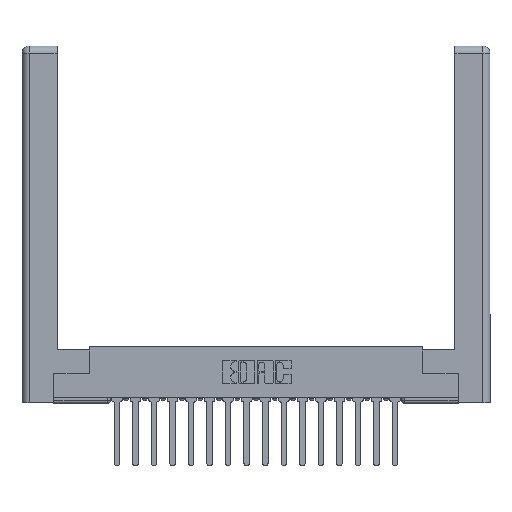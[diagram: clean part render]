
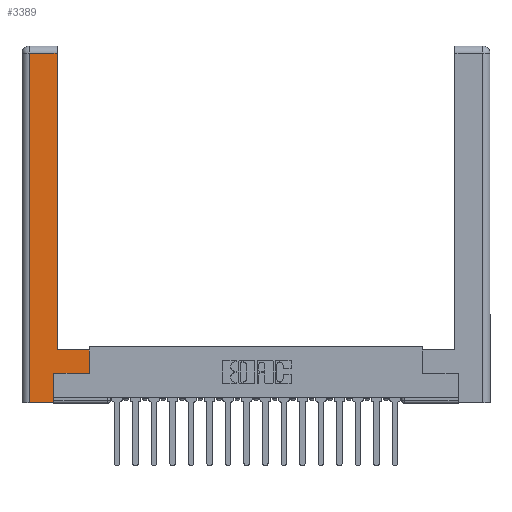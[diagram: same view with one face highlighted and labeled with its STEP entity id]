
A CAD part, top view. The second image highlights one B-rep face of the part: STEP entity #3389.
In plain terms, the highlighted planar face has unit normal (0, 0, 1).
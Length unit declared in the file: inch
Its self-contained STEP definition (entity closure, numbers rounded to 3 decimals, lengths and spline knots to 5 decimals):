
#614 = VECTOR ( 'NONE', #8455, 39.37008 ) ;
#853 = EDGE_CURVE ( 'NONE', #2836, #4499, #2111, .T. ) ;
#856 = EDGE_LOOP ( 'NONE', ( #15141, #6297, #9200, #5167, #18083, #8203, #3710, #19358 ) ) ;
#1286 = DIRECTION ( 'NONE',  ( 0., 1., 0. ) ) ;
#1375 = EDGE_CURVE ( 'NONE', #1869, #11545, #8888, .T. ) ;
#1537 = CARTESIAN_POINT ( 'NONE',  ( 0.565, 0.245, 0. ) ) ;
#1869 = VERTEX_POINT ( 'NONE', #1537 ) ;
#2111 = LINE ( 'NONE', #8160, #614 ) ;
#2508 = CARTESIAN_POINT ( 'NONE',  ( 0.0615, 0., 0. ) ) ;
#2730 = EDGE_CURVE ( 'NONE', #12253, #6543, #13529, .T. ) ;
#2836 = VERTEX_POINT ( 'NONE', #15602 ) ;
#2843 = CARTESIAN_POINT ( 'NONE',  ( 0.565, 0.45, 0. ) ) ;
#2888 = CARTESIAN_POINT ( 'NONE',  ( 0.0615, 2.94, 0. ) ) ;
#3200 = LINE ( 'NONE', #15154, #17868 ) ;
#3276 = EDGE_CURVE ( 'NONE', #8024, #18754, #8373, .T. ) ;
#3389 = ADVANCED_FACE ( 'NONE', ( #11805 ), #5505, .F. ) ;
#3499 = VECTOR ( 'NONE', #13211, 39.37008 ) ;
#3710 = ORIENTED_EDGE ( 'NONE', *, *, #1375, .T. ) ;
#4499 = VERTEX_POINT ( 'NONE', #5431 ) ;
#4807 = DIRECTION ( 'NONE',  ( 1., 0., 0. ) ) ;
#5167 = ORIENTED_EDGE ( 'NONE', *, *, #16092, .T. ) ;
#5282 = CARTESIAN_POINT ( 'NONE',  ( 0.0615, 2.94, 0. ) ) ;
#5431 = CARTESIAN_POINT ( 'NONE',  ( 0.265, 0.245, 0. ) ) ;
#5479 = VECTOR ( 'NONE', #1286, 39.37008 ) ;
#5505 = PLANE ( 'NONE',  #19363 ) ;
#6297 = ORIENTED_EDGE ( 'NONE', *, *, #10881, .T. ) ;
#6543 = VERTEX_POINT ( 'NONE', #16016 ) ;
#7455 = CARTESIAN_POINT ( 'NONE',  ( 0.295, 3., 0. ) ) ;
#7526 = EDGE_CURVE ( 'NONE', #11545, #12253, #13202, .T. ) ;
#8024 = VERTEX_POINT ( 'NONE', #5282 ) ;
#8122 = DIRECTION ( 'NONE',  ( 1., 0., 0. ) ) ;
#8160 = CARTESIAN_POINT ( 'NONE',  ( 0.265, 0.245, 0. ) ) ;
#8203 = ORIENTED_EDGE ( 'NONE', *, *, #19004, .T. ) ;
#8373 = LINE ( 'NONE', #12599, #11798 ) ;
#8455 = DIRECTION ( 'NONE',  ( 0., 1., 0. ) ) ;
#8855 = VECTOR ( 'NONE', #15041, 39.37008 ) ;
#8888 = LINE ( 'NONE', #2843, #3499 ) ;
#9200 = ORIENTED_EDGE ( 'NONE', *, *, #3276, .T. ) ;
#9609 = CARTESIAN_POINT ( 'NONE',  ( 0.295, 0.45, 0. ) ) ;
#10112 = DIRECTION ( 'NONE',  ( -1., 0., 0. ) ) ;
#10156 = CARTESIAN_POINT ( 'NONE',  ( 0.295, 0.45, 0. ) ) ;
#10223 = CARTESIAN_POINT ( 'NONE',  ( 0., 0., 0. ) ) ;
#10576 = VECTOR ( 'NONE', #14580, 39.37008 ) ;
#10881 = EDGE_CURVE ( 'NONE', #6543, #8024, #16418, .T. ) ;
#11545 = VERTEX_POINT ( 'NONE', #17468 ) ;
#11798 = VECTOR ( 'NONE', #14363, 39.37008 ) ;
#11805 = FACE_OUTER_BOUND ( 'NONE', #856, .T. ) ;
#12253 = VERTEX_POINT ( 'NONE', #9609 ) ;
#12599 = CARTESIAN_POINT ( 'NONE',  ( 0.0615, 0., 0. ) ) ;
#12742 = CARTESIAN_POINT ( 'NONE',  ( 0.265, 0., 0. ) ) ;
#13202 = LINE ( 'NONE', #10156, #10576 ) ;
#13211 = DIRECTION ( 'NONE',  ( 0., 1., 0. ) ) ;
#13529 = LINE ( 'NONE', #7455, #5479 ) ;
#14204 = LINE ( 'NONE', #12742, #17138 ) ;
#14363 = DIRECTION ( 'NONE',  ( 0., -1., 0. ) ) ;
#14580 = DIRECTION ( 'NONE',  ( -1., 0., 0. ) ) ;
#14846 = DIRECTION ( 'NONE',  ( 0., 0., -1. ) ) ;
#15041 = DIRECTION ( 'NONE',  ( -1., 0., 0. ) ) ;
#15141 = ORIENTED_EDGE ( 'NONE', *, *, #2730, .T. ) ;
#15154 = CARTESIAN_POINT ( 'NONE',  ( 0.565, 0.245, 0. ) ) ;
#15602 = CARTESIAN_POINT ( 'NONE',  ( 0.265, 0., 0. ) ) ;
#16016 = CARTESIAN_POINT ( 'NONE',  ( 0.295, 2.94, 0. ) ) ;
#16092 = EDGE_CURVE ( 'NONE', #18754, #2836, #14204, .T. ) ;
#16418 = LINE ( 'NONE', #2888, #8855 ) ;
#17138 = VECTOR ( 'NONE', #8122, 39.37008 ) ;
#17468 = CARTESIAN_POINT ( 'NONE',  ( 0.565, 0.45, 0. ) ) ;
#17868 = VECTOR ( 'NONE', #4807, 39.37008 ) ;
#18083 = ORIENTED_EDGE ( 'NONE', *, *, #853, .T. ) ;
#18754 = VERTEX_POINT ( 'NONE', #2508 ) ;
#19004 = EDGE_CURVE ( 'NONE', #4499, #1869, #3200, .T. ) ;
#19358 = ORIENTED_EDGE ( 'NONE', *, *, #7526, .T. ) ;
#19363 = AXIS2_PLACEMENT_3D ( 'NONE', #10223, #14846, #10112 ) ;
